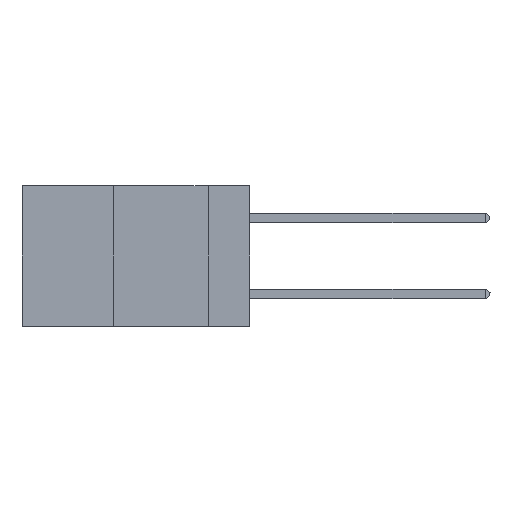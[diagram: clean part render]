
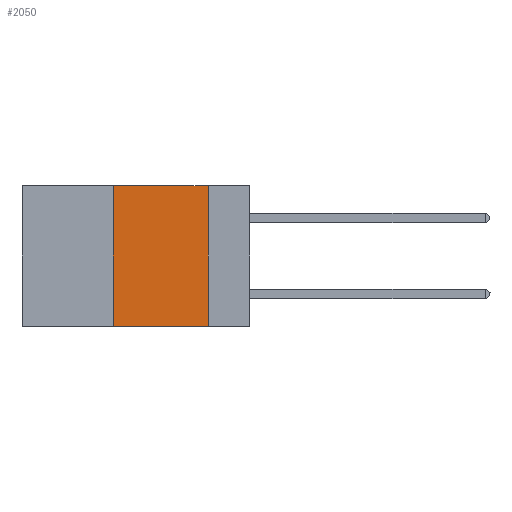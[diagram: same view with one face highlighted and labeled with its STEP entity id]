
A CAD part, left-side view. The second image highlights one B-rep face of the part: STEP entity #2050.
In plain terms, the highlighted planar face has unit normal (-1, 0, 0).
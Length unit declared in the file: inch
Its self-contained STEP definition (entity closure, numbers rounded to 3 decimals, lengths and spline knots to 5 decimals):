
#723 = DIRECTION ( 'NONE',  ( 1., 0., 0. ) ) ;
#770 = VECTOR ( 'NONE', #7745, 39.37008 ) ;
#2050 = ADVANCED_FACE ( 'NONE', ( #9260 ), #18253, .F. ) ;
#2356 = ORIENTED_EDGE ( 'NONE', *, *, #6382, .F. ) ;
#2441 = CARTESIAN_POINT ( 'NONE',  ( 0., 0.11, 0. ) ) ;
#3002 = VECTOR ( 'NONE', #21801, 39.37008 ) ;
#3534 = EDGE_CURVE ( 'NONE', #6857, #8552, #5316, .T. ) ;
#4205 = VERTEX_POINT ( 'NONE', #15352 ) ;
#4820 = CARTESIAN_POINT ( 'NONE',  ( 0., 0.36, -0.37 ) ) ;
#5316 = LINE ( 'NONE', #11399, #10582 ) ;
#5429 = LINE ( 'NONE', #2441, #770 ) ;
#6382 = EDGE_CURVE ( 'NONE', #16514, #6857, #19200, .T. ) ;
#6857 = VERTEX_POINT ( 'NONE', #8068 ) ;
#7745 = DIRECTION ( 'NONE',  ( 0., 0., -1. ) ) ;
#8068 = CARTESIAN_POINT ( 'NONE',  ( 0., 0.36, 0. ) ) ;
#8313 = LINE ( 'NONE', #19584, #16573 ) ;
#8527 = ORIENTED_EDGE ( 'NONE', *, *, #9452, .T. ) ;
#8552 = VERTEX_POINT ( 'NONE', #19971 ) ;
#9260 = FACE_OUTER_BOUND ( 'NONE', #19981, .T. ) ;
#9452 = EDGE_CURVE ( 'NONE', #16514, #4205, #8313, .T. ) ;
#10582 = VECTOR ( 'NONE', #16699, 39.37008 ) ;
#11399 = CARTESIAN_POINT ( 'NONE',  ( 0., 0.6, 0. ) ) ;
#11439 = DIRECTION ( 'NONE',  ( 0., 0., -1. ) ) ;
#12513 = DIRECTION ( 'NONE',  ( 0., -1., 0. ) ) ;
#14282 = AXIS2_PLACEMENT_3D ( 'NONE', #16589, #723, #11439 ) ;
#15352 = CARTESIAN_POINT ( 'NONE',  ( 0., 0.11, -0.37 ) ) ;
#16476 = CARTESIAN_POINT ( 'NONE',  ( 0., 0.36, 0. ) ) ;
#16514 = VERTEX_POINT ( 'NONE', #4820 ) ;
#16573 = VECTOR ( 'NONE', #12513, 39.37008 ) ;
#16589 = CARTESIAN_POINT ( 'NONE',  ( 0., 0.6, 0. ) ) ;
#16699 = DIRECTION ( 'NONE',  ( 0., -1., 0. ) ) ;
#17204 = EDGE_CURVE ( 'NONE', #8552, #4205, #5429, .T. ) ;
#18253 = PLANE ( 'NONE',  #14282 ) ;
#19200 = LINE ( 'NONE', #16476, #3002 ) ;
#19584 = CARTESIAN_POINT ( 'NONE',  ( 0., 0.6, -0.37 ) ) ;
#19971 = CARTESIAN_POINT ( 'NONE',  ( 0., 0.11, 0. ) ) ;
#19981 = EDGE_LOOP ( 'NONE', ( #22005, #21467, #2356, #8527 ) ) ;
#21467 = ORIENTED_EDGE ( 'NONE', *, *, #3534, .F. ) ;
#21801 = DIRECTION ( 'NONE',  ( 0., 0., 1. ) ) ;
#22005 = ORIENTED_EDGE ( 'NONE', *, *, #17204, .F. ) ;
